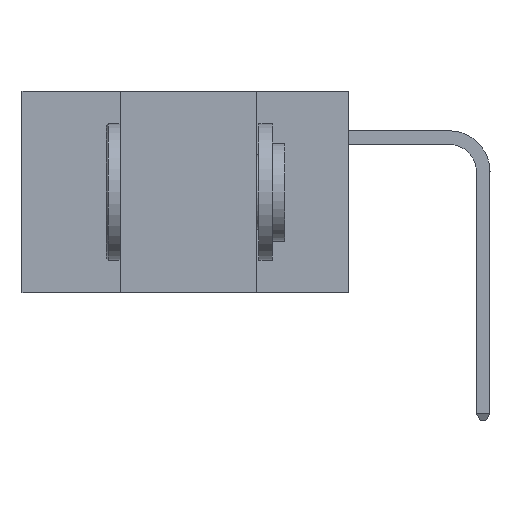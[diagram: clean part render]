
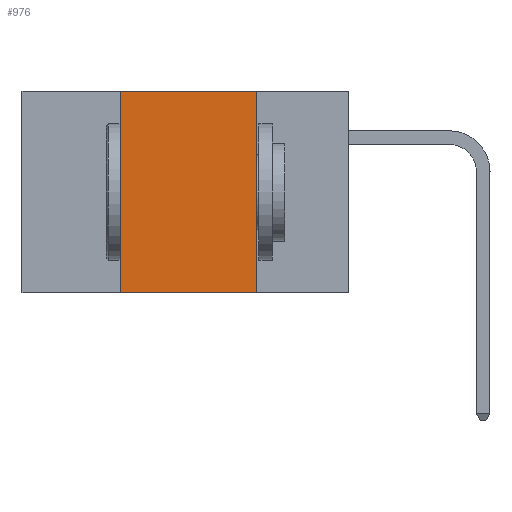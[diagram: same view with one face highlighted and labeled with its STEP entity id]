
A CAD part, left-side view. The second image highlights one B-rep face of the part: STEP entity #976.
In plain terms, the highlighted planar face has unit normal (-1, 0, 0).
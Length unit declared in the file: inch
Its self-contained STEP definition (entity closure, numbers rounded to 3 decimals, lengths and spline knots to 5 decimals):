
#976 = ADVANCED_FACE ( 'NONE', ( #24405 ), #42111, .F. ) ;
#1130 = VERTEX_POINT ( 'NONE', #22743 ) ;
#1157 = DIRECTION ( 'NONE',  ( 0., -1., 0. ) ) ;
#1873 = LINE ( 'NONE', #33871, #34594 ) ;
#1919 = VECTOR ( 'NONE', #1157, 39.37008 ) ;
#3237 = DIRECTION ( 'NONE',  ( 0., 0., -1. ) ) ;
#3796 = VERTEX_POINT ( 'NONE', #28079 ) ;
#5700 = LINE ( 'NONE', #18734, #12327 ) ;
#7249 = VECTOR ( 'NONE', #11282, 39.37008 ) ;
#8141 = CARTESIAN_POINT ( 'NONE',  ( 0., 0.42, 0. ) ) ;
#11282 = DIRECTION ( 'NONE',  ( 0., 0., 1. ) ) ;
#12327 = VECTOR ( 'NONE', #41607, 39.37008 ) ;
#13489 = ORIENTED_EDGE ( 'NONE', *, *, #38078, .F. ) ;
#14699 = LINE ( 'NONE', #24302, #1919 ) ;
#16693 = AXIS2_PLACEMENT_3D ( 'NONE', #22518, #19379, #3237 ) ;
#16958 = CARTESIAN_POINT ( 'NONE',  ( 0., 0.17, -0.37 ) ) ;
#18734 = CARTESIAN_POINT ( 'NONE',  ( 0., 0.6, -0.37 ) ) ;
#19379 = DIRECTION ( 'NONE',  ( 1., 0., 0. ) ) ;
#22518 = CARTESIAN_POINT ( 'NONE',  ( 0., 0.6, 0. ) ) ;
#22743 = CARTESIAN_POINT ( 'NONE',  ( 0., 0.42, -0.37 ) ) ;
#23014 = EDGE_LOOP ( 'NONE', ( #42054, #36150, #13489, #28933 ) ) ;
#23295 = VERTEX_POINT ( 'NONE', #38338 ) ;
#24129 = LINE ( 'NONE', #8141, #7249 ) ;
#24302 = CARTESIAN_POINT ( 'NONE',  ( 0., 0.6, 0. ) ) ;
#24405 = FACE_OUTER_BOUND ( 'NONE', #23014, .T. ) ;
#28079 = CARTESIAN_POINT ( 'NONE',  ( 0., 0.42, 0. ) ) ;
#28933 = ORIENTED_EDGE ( 'NONE', *, *, #30026, .T. ) ;
#30026 = EDGE_CURVE ( 'NONE', #1130, #35835, #5700, .T. ) ;
#31431 = EDGE_CURVE ( 'NONE', #3796, #23295, #14699, .T. ) ;
#32028 = EDGE_CURVE ( 'NONE', #23295, #35835, #1873, .T. ) ;
#33871 = CARTESIAN_POINT ( 'NONE',  ( 0., 0.17, 0. ) ) ;
#34010 = DIRECTION ( 'NONE',  ( 0., 0., -1. ) ) ;
#34594 = VECTOR ( 'NONE', #34010, 39.37008 ) ;
#35835 = VERTEX_POINT ( 'NONE', #16958 ) ;
#36150 = ORIENTED_EDGE ( 'NONE', *, *, #31431, .F. ) ;
#38078 = EDGE_CURVE ( 'NONE', #1130, #3796, #24129, .T. ) ;
#38338 = CARTESIAN_POINT ( 'NONE',  ( 0., 0.17, 0. ) ) ;
#41607 = DIRECTION ( 'NONE',  ( 0., -1., 0. ) ) ;
#42054 = ORIENTED_EDGE ( 'NONE', *, *, #32028, .F. ) ;
#42111 = PLANE ( 'NONE',  #16693 ) ;
